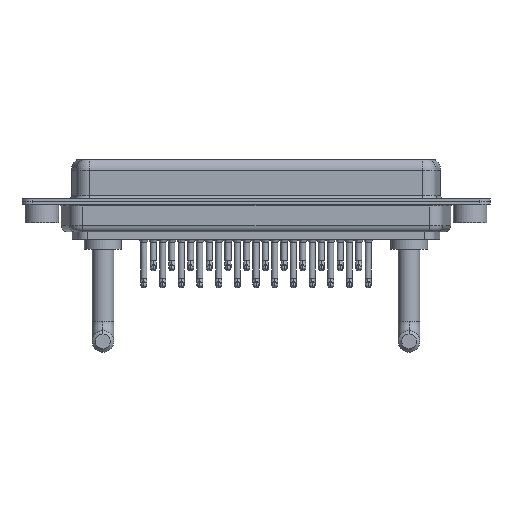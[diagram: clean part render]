
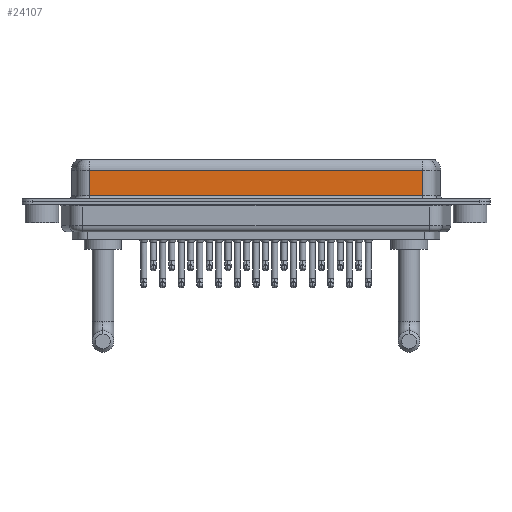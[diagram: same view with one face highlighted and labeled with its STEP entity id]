
A CAD part, front view. The second image highlights one B-rep face of the part: STEP entity #24107.
In plain terms, the highlighted planar face has unit normal (0, -1, 0).
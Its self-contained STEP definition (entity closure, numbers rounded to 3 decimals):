
#746 = DIRECTION ( 'NONE',  ( -1., 0., 0. ) ) ;
#1512 = CARTESIAN_POINT ( 'NONE',  ( 56.462, -3.95, 0.9 ) ) ;
#2038 = DIRECTION ( 'NONE',  ( 1., 0., 0. ) ) ;
#2297 = CARTESIAN_POINT ( 'NONE',  ( 7.038, -3.95, 0.9 ) ) ;
#2481 = FACE_OUTER_BOUND ( 'NONE', #24251, .T. ) ;
#2499 = VERTEX_POINT ( 'NONE', #2297 ) ;
#2743 = DIRECTION ( 'NONE',  ( 0., 0., -1. ) ) ;
#4635 = DIRECTION ( 'NONE',  ( 0., 0., 1. ) ) ;
#8256 = ORIENTED_EDGE ( 'NONE', *, *, #9350, .T. ) ;
#8281 = PLANE ( 'NONE',  #14672 ) ;
#9303 = VECTOR ( 'NONE', #746, 1000. ) ;
#9350 = EDGE_CURVE ( 'NONE', #2499, #9636, #19281, .T. ) ;
#9477 = ORIENTED_EDGE ( 'NONE', *, *, #20378, .F. ) ;
#9636 = VERTEX_POINT ( 'NONE', #1512 ) ;
#11372 = LINE ( 'NONE', #19058, #20108 ) ;
#12780 = ORIENTED_EDGE ( 'NONE', *, *, #21171, .T. ) ;
#12969 = CARTESIAN_POINT ( 'NONE',  ( 56.462, -3.95, 4.65 ) ) ;
#13925 = CARTESIAN_POINT ( 'NONE',  ( 7.038, -3.95, 4.65 ) ) ;
#14192 = CARTESIAN_POINT ( 'NONE',  ( 56.462, -3.95, 6.4 ) ) ;
#14672 = AXIS2_PLACEMENT_3D ( 'NONE', #14192, #21860, #4635 ) ;
#14986 = VERTEX_POINT ( 'NONE', #13925 ) ;
#16477 = LINE ( 'NONE', #20132, #22563 ) ;
#17074 = ORIENTED_EDGE ( 'NONE', *, *, #21090, .T. ) ;
#17298 = VECTOR ( 'NONE', #2038, 1000. ) ;
#17997 = CARTESIAN_POINT ( 'NONE',  ( 56.462, -3.95, 4.65 ) ) ;
#19058 = CARTESIAN_POINT ( 'NONE',  ( 56.462, -3.95, 6.4 ) ) ;
#19281 = LINE ( 'NONE', #23043, #17298 ) ;
#20108 = VECTOR ( 'NONE', #24820, 1000. ) ;
#20132 = CARTESIAN_POINT ( 'NONE',  ( 7.038, -3.95, 6.4 ) ) ;
#20258 = LINE ( 'NONE', #17997, #9303 ) ;
#20378 = EDGE_CURVE ( 'NONE', #22495, #9636, #11372, .T. ) ;
#21090 = EDGE_CURVE ( 'NONE', #14986, #2499, #16477, .T. ) ;
#21171 = EDGE_CURVE ( 'NONE', #22495, #14986, #20258, .T. ) ;
#21860 = DIRECTION ( 'NONE',  ( 0., 1., 0. ) ) ;
#22495 = VERTEX_POINT ( 'NONE', #12969 ) ;
#22563 = VECTOR ( 'NONE', #2743, 1000. ) ;
#23043 = CARTESIAN_POINT ( 'NONE',  ( 56.462, -3.95, 0.9 ) ) ;
#24107 = ADVANCED_FACE ( 'NONE', ( #2481 ), #8281, .F. ) ;
#24251 = EDGE_LOOP ( 'NONE', ( #9477, #12780, #17074, #8256 ) ) ;
#24820 = DIRECTION ( 'NONE',  ( 0., 0., -1. ) ) ;
